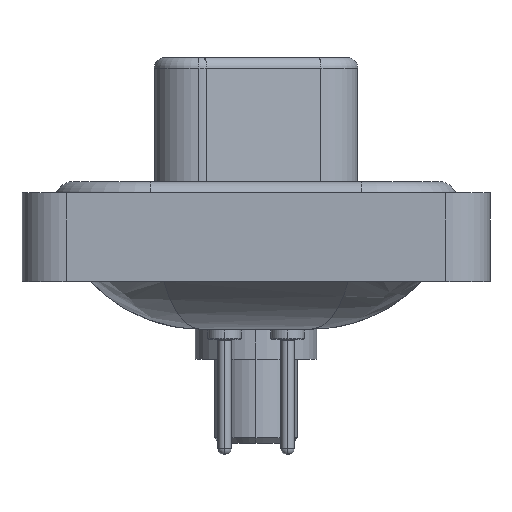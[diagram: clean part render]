
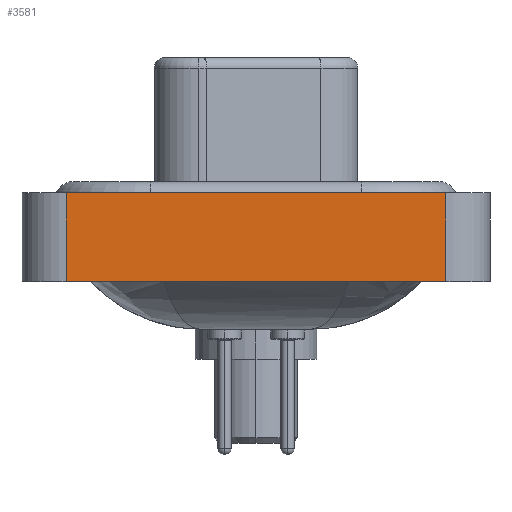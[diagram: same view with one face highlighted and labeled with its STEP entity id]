
A CAD part, left-side view. The second image highlights one B-rep face of the part: STEP entity #3581.
In plain terms, the highlighted planar face has unit normal (-1, 0, 0).
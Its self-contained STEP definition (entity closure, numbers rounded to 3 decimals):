
#1731 = EDGE_CURVE ( 'NONE', #9981, #21481, #13943, .T. ) ;
#2469 = DIRECTION ( 'NONE',  ( -1., 0., 0. ) ) ;
#2587 = ORIENTED_EDGE ( 'NONE', *, *, #20721, .F. ) ;
#2683 = DIRECTION ( 'NONE',  ( 0., 0., 1. ) ) ;
#3581 = ADVANCED_FACE ( 'NONE', ( #22489 ), #13473, .T. ) ;
#3803 = CARTESIAN_POINT ( 'NONE',  ( -7.35, -8.55, -3.6 ) ) ;
#4549 = VERTEX_POINT ( 'NONE', #6040 ) ;
#5528 = CARTESIAN_POINT ( 'NONE',  ( -7.35, -8.55, -3.6 ) ) ;
#5552 = VERTEX_POINT ( 'NONE', #21476 ) ;
#6040 = CARTESIAN_POINT ( 'NONE',  ( -7.35, 8.55, -3.6 ) ) ;
#6108 = CARTESIAN_POINT ( 'NONE',  ( -7.35, -8.55, -3.6 ) ) ;
#7944 = VECTOR ( 'NONE', #10270, 1000. ) ;
#9009 = CARTESIAN_POINT ( 'NONE',  ( -7.35, -8.55, -3.6 ) ) ;
#9671 = DIRECTION ( 'NONE',  ( 0., 0., 1. ) ) ;
#9981 = VERTEX_POINT ( 'NONE', #5528 ) ;
#10270 = DIRECTION ( 'NONE',  ( 0., 0., 1. ) ) ;
#10639 = LINE ( 'NONE', #18086, #13650 ) ;
#11905 = VECTOR ( 'NONE', #2683, 1000. ) ;
#13324 = EDGE_CURVE ( 'NONE', #4549, #9981, #20110, .T. ) ;
#13473 = PLANE ( 'NONE',  #13580 ) ;
#13580 = AXIS2_PLACEMENT_3D ( 'NONE', #3803, #2469, #9671 ) ;
#13650 = VECTOR ( 'NONE', #16697, 1000. ) ;
#13742 = ORIENTED_EDGE ( 'NONE', *, *, #13324, .T. ) ;
#13801 = EDGE_LOOP ( 'NONE', ( #14970, #2587, #16798, #13742 ) ) ;
#13827 = LINE ( 'NONE', #20997, #7944 ) ;
#13943 = LINE ( 'NONE', #6108, #11905 ) ;
#13991 = EDGE_CURVE ( 'NONE', #4549, #5552, #13827, .T. ) ;
#14970 = ORIENTED_EDGE ( 'NONE', *, *, #1731, .T. ) ;
#15258 = VECTOR ( 'NONE', #18767, 1000. ) ;
#16697 = DIRECTION ( 'NONE',  ( 0., -1., 0. ) ) ;
#16798 = ORIENTED_EDGE ( 'NONE', *, *, #13991, .F. ) ;
#18086 = CARTESIAN_POINT ( 'NONE',  ( -7.35, -8.55, 0.4 ) ) ;
#18351 = CARTESIAN_POINT ( 'NONE',  ( -7.35, -8.55, 0.4 ) ) ;
#18767 = DIRECTION ( 'NONE',  ( 0., -1., 0. ) ) ;
#20110 = LINE ( 'NONE', #9009, #15258 ) ;
#20721 = EDGE_CURVE ( 'NONE', #5552, #21481, #10639, .T. ) ;
#20997 = CARTESIAN_POINT ( 'NONE',  ( -7.35, 8.55, -3.6 ) ) ;
#21476 = CARTESIAN_POINT ( 'NONE',  ( -7.35, 8.55, 0.4 ) ) ;
#21481 = VERTEX_POINT ( 'NONE', #18351 ) ;
#22489 = FACE_OUTER_BOUND ( 'NONE', #13801, .T. ) ;
